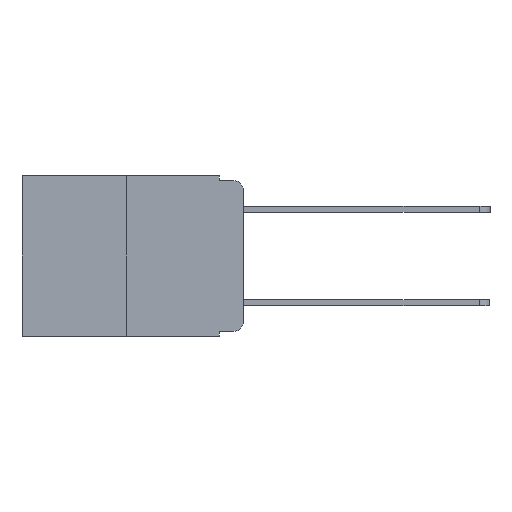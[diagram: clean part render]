
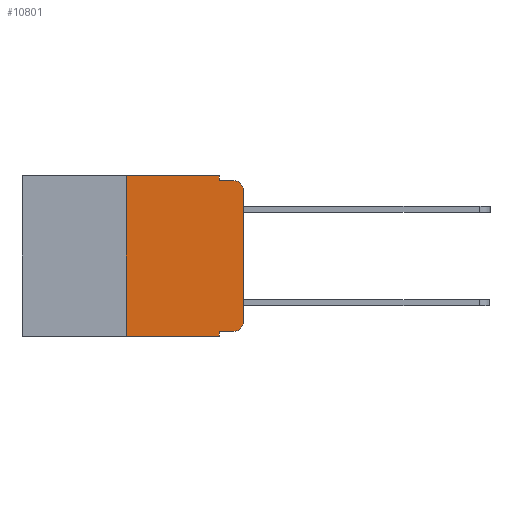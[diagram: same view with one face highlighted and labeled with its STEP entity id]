
A CAD part, left-side view. The second image highlights one B-rep face of the part: STEP entity #10801.
In plain terms, the highlighted planar face has unit normal (-1, 0, 0).
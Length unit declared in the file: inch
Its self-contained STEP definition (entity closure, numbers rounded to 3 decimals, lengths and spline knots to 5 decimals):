
#436 = ORIENTED_EDGE ( 'NONE', *, *, #13531, .F. ) ;
#514 = CARTESIAN_POINT ( 'NONE',  ( 0., 0.25, 0. ) ) ;
#658 = CARTESIAN_POINT ( 'NONE',  ( 0., 0.02, -0.03 ) ) ;
#715 = EDGE_CURVE ( 'NONE', #17392, #12564, #13432, .T. ) ;
#726 = VECTOR ( 'NONE', #13542, 39.37008 ) ;
#2012 = CARTESIAN_POINT ( 'NONE',  ( 0., 0.051, 0. ) ) ;
#2066 = VERTEX_POINT ( 'NONE', #13365 ) ;
#2118 = VERTEX_POINT ( 'NONE', #11478 ) ;
#2252 = LINE ( 'NONE', #10659, #15524 ) ;
#2281 = ORIENTED_EDGE ( 'NONE', *, *, #715, .F. ) ;
#2345 = DIRECTION ( 'NONE',  ( 0., 0., -1. ) ) ;
#3016 = EDGE_CURVE ( 'NONE', #12564, #4424, #21502, .T. ) ;
#3153 = CARTESIAN_POINT ( 'NONE',  ( 0., 0.02, -0.333 ) ) ;
#3653 = VECTOR ( 'NONE', #7134, 39.37008 ) ;
#4424 = VERTEX_POINT ( 'NONE', #4866 ) ;
#4866 = CARTESIAN_POINT ( 'NONE',  ( 0., 0.02, -0.01 ) ) ;
#4905 = CARTESIAN_POINT ( 'NONE',  ( 0., 0.25, -0.343 ) ) ;
#4920 = LINE ( 'NONE', #10903, #21551 ) ;
#5465 = DIRECTION ( 'NONE',  ( 0., 0., -1. ) ) ;
#5834 = VERTEX_POINT ( 'NONE', #8476 ) ;
#6082 = AXIS2_PLACEMENT_3D ( 'NONE', #8086, #19790, #9777 ) ;
#6340 = AXIS2_PLACEMENT_3D ( 'NONE', #7029, #15395, #5465 ) ;
#6918 = EDGE_LOOP ( 'NONE', ( #21569, #11384, #20777, #2281, #436, #11357, #18957, #7489, #18442, #11362 ) ) ;
#7029 = CARTESIAN_POINT ( 'NONE',  ( 0., 0.473, 0. ) ) ;
#7134 = DIRECTION ( 'NONE',  ( 0., 0., 1. ) ) ;
#7180 = VECTOR ( 'NONE', #9222, 39.37008 ) ;
#7489 = ORIENTED_EDGE ( 'NONE', *, *, #12022, .F. ) ;
#7557 = CARTESIAN_POINT ( 'NONE',  ( 0., 0.051, -0.333 ) ) ;
#8086 = CARTESIAN_POINT ( 'NONE',  ( 0., 0.02, -0.313 ) ) ;
#8375 = EDGE_CURVE ( 'NONE', #21543, #2066, #12401, .T. ) ;
#8476 = CARTESIAN_POINT ( 'NONE',  ( 0., 0.051, -0.343 ) ) ;
#8729 = VERTEX_POINT ( 'NONE', #3153 ) ;
#9222 = DIRECTION ( 'NONE',  ( 0., -1., 0. ) ) ;
#9576 = DIRECTION ( 'NONE',  ( 0., 0., 1. ) ) ;
#9777 = DIRECTION ( 'NONE',  ( 0., 0., -1. ) ) ;
#10375 = VECTOR ( 'NONE', #9576, 39.37008 ) ;
#10659 = CARTESIAN_POINT ( 'NONE',  ( 0., 0.473, 0. ) ) ;
#10759 = CARTESIAN_POINT ( 'NONE',  ( 0., 0., -0.313 ) ) ;
#10801 = ADVANCED_FACE ( 'NONE', ( #11190 ), #12002, .F. ) ;
#10895 = LINE ( 'NONE', #11217, #10375 ) ;
#10903 = CARTESIAN_POINT ( 'NONE',  ( 0., 0.473, -0.343 ) ) ;
#11190 = FACE_OUTER_BOUND ( 'NONE', #6918, .T. ) ;
#11217 = CARTESIAN_POINT ( 'NONE',  ( 0., 0.25, 0. ) ) ;
#11357 = ORIENTED_EDGE ( 'NONE', *, *, #11935, .F. ) ;
#11362 = ORIENTED_EDGE ( 'NONE', *, *, #12510, .T. ) ;
#11384 = ORIENTED_EDGE ( 'NONE', *, *, #18112, .T. ) ;
#11478 = CARTESIAN_POINT ( 'NONE',  ( 0., 0.051, -0.333 ) ) ;
#11935 = EDGE_CURVE ( 'NONE', #20559, #21420, #10895, .T. ) ;
#12002 = PLANE ( 'NONE',  #6340 ) ;
#12022 = EDGE_CURVE ( 'NONE', #2118, #5834, #17725, .T. ) ;
#12252 = DIRECTION ( 'NONE',  ( -1., 0., 0. ) ) ;
#12401 = LINE ( 'NONE', #17159, #3653 ) ;
#12510 = EDGE_CURVE ( 'NONE', #8729, #21543, #17701, .T. ) ;
#12564 = VERTEX_POINT ( 'NONE', #18242 ) ;
#12974 = EDGE_CURVE ( 'NONE', #20559, #5834, #4920, .T. ) ;
#13192 = VECTOR ( 'NONE', #21449, 39.37008 ) ;
#13365 = CARTESIAN_POINT ( 'NONE',  ( 0., 0., -0.03 ) ) ;
#13414 = CARTESIAN_POINT ( 'NONE',  ( 0., 0.051, 0. ) ) ;
#13432 = LINE ( 'NONE', #13414, #726 ) ;
#13531 = EDGE_CURVE ( 'NONE', #21420, #17392, #2252, .T. ) ;
#13542 = DIRECTION ( 'NONE',  ( 0., 0., -1. ) ) ;
#14391 = CIRCLE ( 'NONE', #15532, 0.02 ) ;
#15395 = DIRECTION ( 'NONE',  ( 1., 0., 0. ) ) ;
#15524 = VECTOR ( 'NONE', #20663, 39.37008 ) ;
#15532 = AXIS2_PLACEMENT_3D ( 'NONE', #658, #12252, #2345 ) ;
#16566 = EDGE_CURVE ( 'NONE', #2118, #8729, #18919, .T. ) ;
#17096 = VECTOR ( 'NONE', #19131, 39.37008 ) ;
#17159 = CARTESIAN_POINT ( 'NONE',  ( 0., 0., 0. ) ) ;
#17392 = VERTEX_POINT ( 'NONE', #2012 ) ;
#17701 = CIRCLE ( 'NONE', #6082, 0.02 ) ;
#17725 = LINE ( 'NONE', #18116, #13192 ) ;
#18112 = EDGE_CURVE ( 'NONE', #2066, #4424, #14391, .T. ) ;
#18116 = CARTESIAN_POINT ( 'NONE',  ( 0., 0.051, 0. ) ) ;
#18242 = CARTESIAN_POINT ( 'NONE',  ( 0., 0.051, -0.01 ) ) ;
#18392 = CARTESIAN_POINT ( 'NONE',  ( 0., 0.051, -0.01 ) ) ;
#18442 = ORIENTED_EDGE ( 'NONE', *, *, #16566, .T. ) ;
#18919 = LINE ( 'NONE', #7557, #7180 ) ;
#18957 = ORIENTED_EDGE ( 'NONE', *, *, #12974, .T. ) ;
#19131 = DIRECTION ( 'NONE',  ( 0., -1., 0. ) ) ;
#19790 = DIRECTION ( 'NONE',  ( -1., 0., 0. ) ) ;
#20559 = VERTEX_POINT ( 'NONE', #4905 ) ;
#20663 = DIRECTION ( 'NONE',  ( 0., -1., 0. ) ) ;
#20777 = ORIENTED_EDGE ( 'NONE', *, *, #3016, .F. ) ;
#20900 = DIRECTION ( 'NONE',  ( 0., -1., 0. ) ) ;
#21420 = VERTEX_POINT ( 'NONE', #514 ) ;
#21449 = DIRECTION ( 'NONE',  ( 0., 0., -1. ) ) ;
#21502 = LINE ( 'NONE', #18392, #17096 ) ;
#21543 = VERTEX_POINT ( 'NONE', #10759 ) ;
#21551 = VECTOR ( 'NONE', #20900, 39.37008 ) ;
#21569 = ORIENTED_EDGE ( 'NONE', *, *, #8375, .T. ) ;
